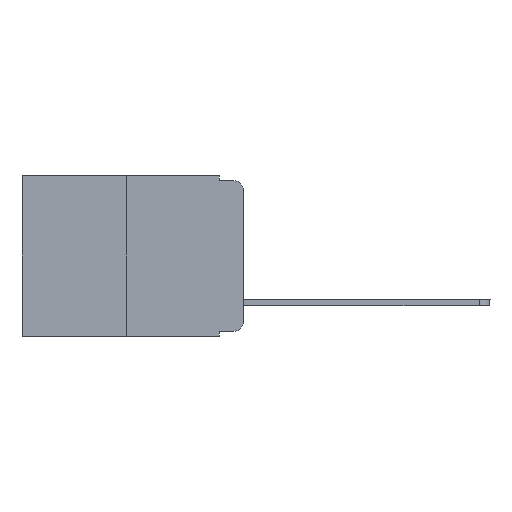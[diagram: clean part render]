
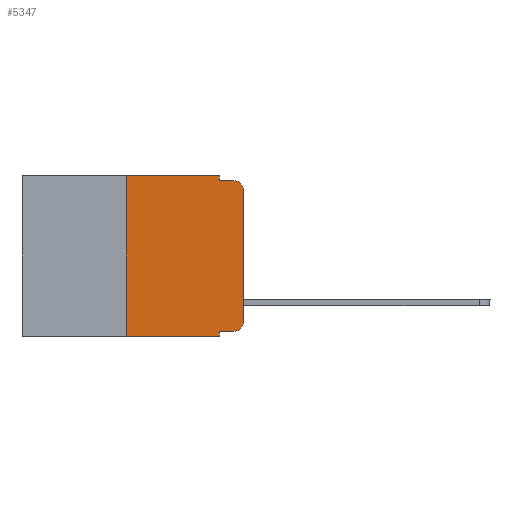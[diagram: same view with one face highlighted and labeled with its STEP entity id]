
A CAD part, left-side view. The second image highlights one B-rep face of the part: STEP entity #5347.
In plain terms, the highlighted planar face has unit normal (-1, 0, 0).
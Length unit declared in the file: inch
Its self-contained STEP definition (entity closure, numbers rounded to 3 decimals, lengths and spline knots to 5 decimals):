
#52 = DIRECTION ( 'NONE',  ( 0., 0., -1. ) ) ;
#235 = LINE ( 'NONE', #11824, #6296 ) ;
#394 = VECTOR ( 'NONE', #14487, 39.37008 ) ;
#597 = CARTESIAN_POINT ( 'NONE',  ( 0., 0.473, 0. ) ) ;
#633 = EDGE_CURVE ( 'NONE', #15107, #13045, #19221, .T. ) ;
#1328 = DIRECTION ( 'NONE',  ( 0., -1., 0. ) ) ;
#1810 = CARTESIAN_POINT ( 'NONE',  ( 0., 0.051, -0.333 ) ) ;
#1952 = DIRECTION ( 'NONE',  ( 0., 0., 1. ) ) ;
#2147 = DIRECTION ( 'NONE',  ( 1., 0., 0. ) ) ;
#2468 = CARTESIAN_POINT ( 'NONE',  ( 0., 0.25, 0. ) ) ;
#2667 = LINE ( 'NONE', #9390, #5299 ) ;
#2871 = EDGE_CURVE ( 'NONE', #10966, #13045, #15749, .T. ) ;
#2989 = DIRECTION ( 'NONE',  ( 0., -1., 0. ) ) ;
#3612 = CARTESIAN_POINT ( 'NONE',  ( 0., 0.25, 0. ) ) ;
#3784 = EDGE_CURVE ( 'NONE', #15107, #19557, #15450, .T. ) ;
#4117 = VERTEX_POINT ( 'NONE', #13707 ) ;
#4280 = CARTESIAN_POINT ( 'NONE',  ( 0., 0.02, -0.313 ) ) ;
#4864 = ORIENTED_EDGE ( 'NONE', *, *, #633, .F. ) ;
#5076 = CARTESIAN_POINT ( 'NONE',  ( 0., 0.051, 0. ) ) ;
#5091 = ORIENTED_EDGE ( 'NONE', *, *, #18510, .F. ) ;
#5207 = VECTOR ( 'NONE', #12166, 39.37008 ) ;
#5299 = VECTOR ( 'NONE', #2989, 39.37008 ) ;
#5304 = VERTEX_POINT ( 'NONE', #10531 ) ;
#5347 = ADVANCED_FACE ( 'NONE', ( #8658 ), #15676, .F. ) ;
#5351 = LINE ( 'NONE', #2468, #20442 ) ;
#5624 = ORIENTED_EDGE ( 'NONE', *, *, #2871, .T. ) ;
#5691 = ORIENTED_EDGE ( 'NONE', *, *, #15002, .T. ) ;
#6296 = VECTOR ( 'NONE', #18623, 39.37008 ) ;
#6330 = EDGE_CURVE ( 'NONE', #5304, #4117, #10418, .T. ) ;
#6560 = DIRECTION ( 'NONE',  ( -1., 0., 0. ) ) ;
#6563 = ORIENTED_EDGE ( 'NONE', *, *, #20818, .T. ) ;
#6664 = AXIS2_PLACEMENT_3D ( 'NONE', #4280, #6560, #14394 ) ;
#6689 = CARTESIAN_POINT ( 'NONE',  ( 0., 0.02, -0.333 ) ) ;
#7030 = CARTESIAN_POINT ( 'NONE',  ( 0., 0., 0. ) ) ;
#7724 = ORIENTED_EDGE ( 'NONE', *, *, #14194, .F. ) ;
#7978 = ORIENTED_EDGE ( 'NONE', *, *, #13786, .F. ) ;
#8085 = CIRCLE ( 'NONE', #6664, 0.02 ) ;
#8248 = CARTESIAN_POINT ( 'NONE',  ( 0., 0.02, -0.03 ) ) ;
#8658 = FACE_OUTER_BOUND ( 'NONE', #11493, .T. ) ;
#8692 = VECTOR ( 'NONE', #52, 39.37008 ) ;
#9390 = CARTESIAN_POINT ( 'NONE',  ( 0., 0.051, -0.01 ) ) ;
#9678 = CARTESIAN_POINT ( 'NONE',  ( 0., 0., -0.313 ) ) ;
#10308 = LINE ( 'NONE', #16882, #8692 ) ;
#10418 = CIRCLE ( 'NONE', #10768, 0.02 ) ;
#10531 = CARTESIAN_POINT ( 'NONE',  ( 0., 0., -0.03 ) ) ;
#10753 = DIRECTION ( 'NONE',  ( 0., 0., 1. ) ) ;
#10768 = AXIS2_PLACEMENT_3D ( 'NONE', #8248, #18349, #18563 ) ;
#10966 = VERTEX_POINT ( 'NONE', #20427 ) ;
#11214 = ORIENTED_EDGE ( 'NONE', *, *, #6330, .T. ) ;
#11343 = AXIS2_PLACEMENT_3D ( 'NONE', #597, #2147, #15463 ) ;
#11493 = EDGE_LOOP ( 'NONE', ( #6563, #11214, #5091, #7978, #7724, #20624, #5624, #4864, #18835, #5691 ) ) ;
#11824 = CARTESIAN_POINT ( 'NONE',  ( 0., 0.473, 0. ) ) ;
#12166 = DIRECTION ( 'NONE',  ( 0., -1., 0. ) ) ;
#12539 = CARTESIAN_POINT ( 'NONE',  ( 0., 0.051, -0.343 ) ) ;
#13045 = VERTEX_POINT ( 'NONE', #12539 ) ;
#13175 = CARTESIAN_POINT ( 'NONE',  ( 0., 0.051, -0.01 ) ) ;
#13314 = VERTEX_POINT ( 'NONE', #9678 ) ;
#13628 = LINE ( 'NONE', #7030, #21522 ) ;
#13707 = CARTESIAN_POINT ( 'NONE',  ( 0., 0.02, -0.01 ) ) ;
#13786 = EDGE_CURVE ( 'NONE', #14661, #16469, #10308, .T. ) ;
#14194 = EDGE_CURVE ( 'NONE', #15995, #14661, #235, .T. ) ;
#14372 = CARTESIAN_POINT ( 'NONE',  ( 0., 0.051, 0. ) ) ;
#14394 = DIRECTION ( 'NONE',  ( 0., 0., -1. ) ) ;
#14487 = DIRECTION ( 'NONE',  ( 0., 0., -1. ) ) ;
#14661 = VERTEX_POINT ( 'NONE', #5076 ) ;
#15002 = EDGE_CURVE ( 'NONE', #19557, #13314, #8085, .T. ) ;
#15107 = VERTEX_POINT ( 'NONE', #1810 ) ;
#15343 = CARTESIAN_POINT ( 'NONE',  ( 0., 0.051, -0.333 ) ) ;
#15450 = LINE ( 'NONE', #15343, #5207 ) ;
#15463 = DIRECTION ( 'NONE',  ( 0., 0., -1. ) ) ;
#15676 = PLANE ( 'NONE',  #11343 ) ;
#15749 = LINE ( 'NONE', #21354, #21528 ) ;
#15995 = VERTEX_POINT ( 'NONE', #3612 ) ;
#16469 = VERTEX_POINT ( 'NONE', #13175 ) ;
#16670 = EDGE_CURVE ( 'NONE', #10966, #15995, #5351, .T. ) ;
#16882 = CARTESIAN_POINT ( 'NONE',  ( 0., 0.051, 0. ) ) ;
#18349 = DIRECTION ( 'NONE',  ( -1., 0., 0. ) ) ;
#18510 = EDGE_CURVE ( 'NONE', #16469, #4117, #2667, .T. ) ;
#18563 = DIRECTION ( 'NONE',  ( 0., 0., -1. ) ) ;
#18623 = DIRECTION ( 'NONE',  ( 0., -1., 0. ) ) ;
#18835 = ORIENTED_EDGE ( 'NONE', *, *, #3784, .T. ) ;
#19221 = LINE ( 'NONE', #14372, #394 ) ;
#19557 = VERTEX_POINT ( 'NONE', #6689 ) ;
#20427 = CARTESIAN_POINT ( 'NONE',  ( 0., 0.25, -0.343 ) ) ;
#20442 = VECTOR ( 'NONE', #10753, 39.37008 ) ;
#20624 = ORIENTED_EDGE ( 'NONE', *, *, #16670, .F. ) ;
#20818 = EDGE_CURVE ( 'NONE', #13314, #5304, #13628, .T. ) ;
#21354 = CARTESIAN_POINT ( 'NONE',  ( 0., 0.473, -0.343 ) ) ;
#21522 = VECTOR ( 'NONE', #1952, 39.37008 ) ;
#21528 = VECTOR ( 'NONE', #1328, 39.37008 ) ;
